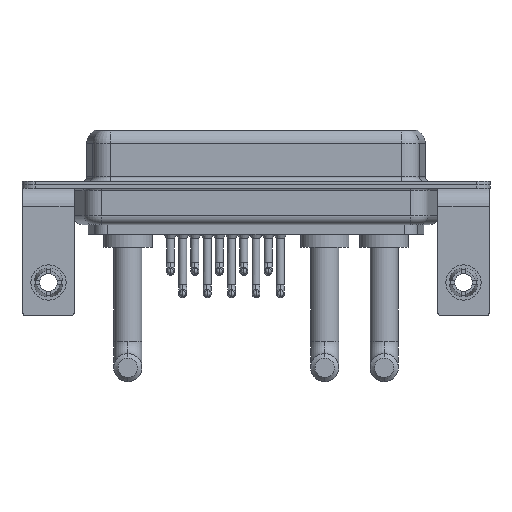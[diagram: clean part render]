
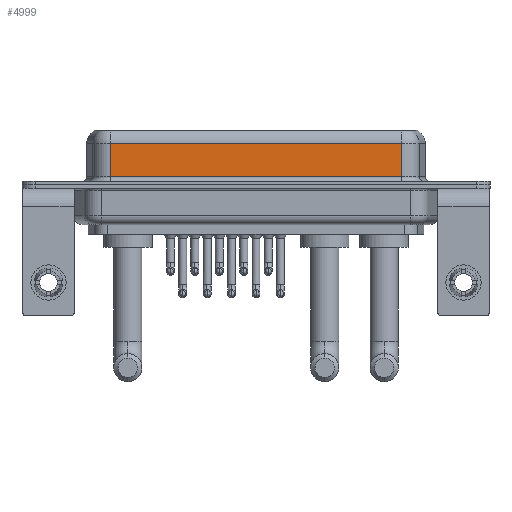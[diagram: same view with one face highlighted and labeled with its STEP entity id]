
A CAD part, front view. The second image highlights one B-rep face of the part: STEP entity #4999.
In plain terms, the highlighted planar face has unit normal (0, -1, 0).
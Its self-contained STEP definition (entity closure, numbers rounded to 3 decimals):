
#584 = FACE_OUTER_BOUND ( 'NONE', #3397, .T. ) ;
#641 = CARTESIAN_POINT ( 'NONE',  ( 7.013, -3.95, 4.65 ) ) ;
#866 = ORIENTED_EDGE ( 'NONE', *, *, #3589, .T. ) ;
#1311 = DIRECTION ( 'NONE',  ( 0., 0., -1. ) ) ;
#1427 = CARTESIAN_POINT ( 'NONE',  ( 40.037, -3.95, 4.65 ) ) ;
#2209 = VECTOR ( 'NONE', #13636, 1000. ) ;
#2222 = CARTESIAN_POINT ( 'NONE',  ( 40.037, -3.95, 0.9 ) ) ;
#2366 = AXIS2_PLACEMENT_3D ( 'NONE', #4287, #17296, #12287 ) ;
#2601 = DIRECTION ( 'NONE',  ( -1., 0., 0. ) ) ;
#3397 = EDGE_LOOP ( 'NONE', ( #13824, #12295, #13579, #866 ) ) ;
#3589 = EDGE_CURVE ( 'NONE', #19383, #20088, #17182, .T. ) ;
#4287 = CARTESIAN_POINT ( 'NONE',  ( 40.037, -3.95, 6.4 ) ) ;
#4577 = CARTESIAN_POINT ( 'NONE',  ( 7.013, -3.95, 6.4 ) ) ;
#4999 = ADVANCED_FACE ( 'NONE', ( #584 ), #12183, .F. ) ;
#5648 = EDGE_CURVE ( 'NONE', #5880, #19383, #19425, .T. ) ;
#5880 = VERTEX_POINT ( 'NONE', #641 ) ;
#8776 = CARTESIAN_POINT ( 'NONE',  ( 40.037, -3.95, 0.9 ) ) ;
#9467 = EDGE_CURVE ( 'NONE', #16131, #5880, #19405, .T. ) ;
#10619 = CARTESIAN_POINT ( 'NONE',  ( 40.037, -3.95, 4.65 ) ) ;
#11636 = EDGE_CURVE ( 'NONE', #16131, #20088, #11896, .T. ) ;
#11720 = VECTOR ( 'NONE', #1311, 1000. ) ;
#11726 = VECTOR ( 'NONE', #15790, 1000. ) ;
#11896 = LINE ( 'NONE', #18616, #2209 ) ;
#12183 = PLANE ( 'NONE',  #2366 ) ;
#12287 = DIRECTION ( 'NONE',  ( 0., 0., 1. ) ) ;
#12295 = ORIENTED_EDGE ( 'NONE', *, *, #9467, .T. ) ;
#13579 = ORIENTED_EDGE ( 'NONE', *, *, #5648, .T. ) ;
#13636 = DIRECTION ( 'NONE',  ( 0., 0., -1. ) ) ;
#13824 = ORIENTED_EDGE ( 'NONE', *, *, #11636, .F. ) ;
#15790 = DIRECTION ( 'NONE',  ( 1., 0., 0. ) ) ;
#16131 = VERTEX_POINT ( 'NONE', #1427 ) ;
#17182 = LINE ( 'NONE', #2222, #11726 ) ;
#17296 = DIRECTION ( 'NONE',  ( 0., 1., 0. ) ) ;
#18616 = CARTESIAN_POINT ( 'NONE',  ( 40.037, -3.95, 6.4 ) ) ;
#18794 = VECTOR ( 'NONE', #2601, 1000. ) ;
#19363 = CARTESIAN_POINT ( 'NONE',  ( 7.013, -3.95, 0.9 ) ) ;
#19383 = VERTEX_POINT ( 'NONE', #19363 ) ;
#19405 = LINE ( 'NONE', #10619, #18794 ) ;
#19425 = LINE ( 'NONE', #4577, #11720 ) ;
#20088 = VERTEX_POINT ( 'NONE', #8776 ) ;
